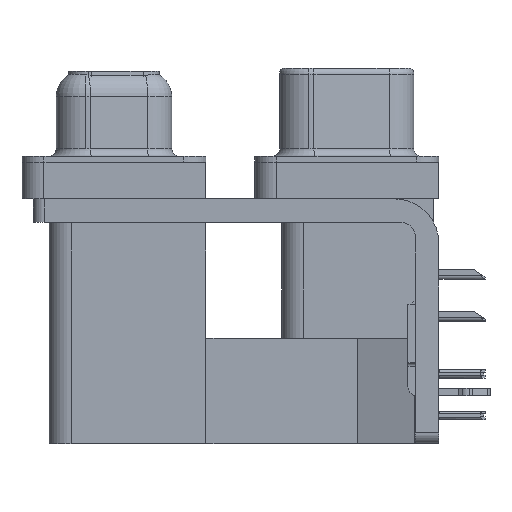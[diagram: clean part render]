
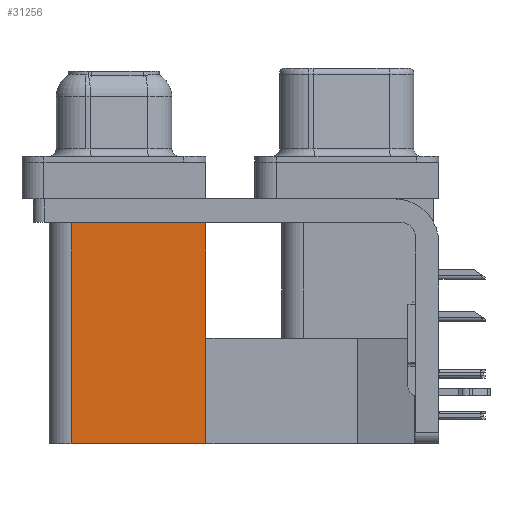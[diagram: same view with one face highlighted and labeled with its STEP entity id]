
A CAD part, left-side view. The second image highlights one B-rep face of the part: STEP entity #31256.
In plain terms, the highlighted planar face has unit normal (-1, 0, 0).
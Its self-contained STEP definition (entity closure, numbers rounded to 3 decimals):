
#248 = AXIS2_PLACEMENT_3D ( 'NONE', #3886, #31192, #4079 ) ;
#544 = CARTESIAN_POINT ( 'NONE',  ( 3.79, 18.8, -19.2 ) ) ;
#741 = CARTESIAN_POINT ( 'NONE',  ( 3.79, 9.6, -2.5 ) ) ;
#758 = CARTESIAN_POINT ( 'NONE',  ( 3.79, 18.8, -2.5 ) ) ;
#1249 = VECTOR ( 'NONE', #10169, 1000. ) ;
#1375 = EDGE_CURVE ( 'NONE', #37500, #7549, #36709, .T. ) ;
#1612 = EDGE_CURVE ( 'NONE', #25228, #7549, #31008, .T. ) ;
#3884 = DIRECTION ( 'NONE',  ( 0., 1., 0. ) ) ;
#3886 = CARTESIAN_POINT ( 'NONE',  ( 3.79, 9.6, -19.2 ) ) ;
#4079 = DIRECTION ( 'NONE',  ( 0., 1., 0. ) ) ;
#6852 = FACE_OUTER_BOUND ( 'NONE', #30425, .T. ) ;
#7549 = VERTEX_POINT ( 'NONE', #758 ) ;
#10169 = DIRECTION ( 'NONE',  ( 0., 0., 1. ) ) ;
#12331 = VECTOR ( 'NONE', #37831, 1000. ) ;
#12776 = ORIENTED_EDGE ( 'NONE', *, *, #1375, .F. ) ;
#14203 = CARTESIAN_POINT ( 'NONE',  ( 3.79, 9.6, -19.2 ) ) ;
#15921 = CARTESIAN_POINT ( 'NONE',  ( 3.79, 18.8, -19.2 ) ) ;
#16997 = VERTEX_POINT ( 'NONE', #14203 ) ;
#18748 = LINE ( 'NONE', #33981, #31999 ) ;
#19130 = DIRECTION ( 'NONE',  ( 0., 1., 0. ) ) ;
#22229 = ORIENTED_EDGE ( 'NONE', *, *, #36298, .F. ) ;
#23211 = ORIENTED_EDGE ( 'NONE', *, *, #27570, .T. ) ;
#25228 = VERTEX_POINT ( 'NONE', #37923 ) ;
#25776 = LINE ( 'NONE', #37448, #12331 ) ;
#27570 = EDGE_CURVE ( 'NONE', #16997, #25228, #25776, .T. ) ;
#30425 = EDGE_LOOP ( 'NONE', ( #32935, #12776, #22229, #23211 ) ) ;
#31008 = LINE ( 'NONE', #741, #32194 ) ;
#31192 = DIRECTION ( 'NONE',  ( 1., 0., 0. ) ) ;
#31256 = ADVANCED_FACE ( 'NONE', ( #6852 ), #37702, .F. ) ;
#31999 = VECTOR ( 'NONE', #19130, 1000. ) ;
#32194 = VECTOR ( 'NONE', #3884, 1000. ) ;
#32935 = ORIENTED_EDGE ( 'NONE', *, *, #1612, .T. ) ;
#33981 = CARTESIAN_POINT ( 'NONE',  ( 3.79, 9.6, -19.2 ) ) ;
#36298 = EDGE_CURVE ( 'NONE', #16997, #37500, #18748, .T. ) ;
#36709 = LINE ( 'NONE', #15921, #1249 ) ;
#37448 = CARTESIAN_POINT ( 'NONE',  ( 3.79, 9.6, -19.2 ) ) ;
#37500 = VERTEX_POINT ( 'NONE', #544 ) ;
#37702 = PLANE ( 'NONE',  #248 ) ;
#37831 = DIRECTION ( 'NONE',  ( 0., 0., 1. ) ) ;
#37923 = CARTESIAN_POINT ( 'NONE',  ( 3.79, 9.6, -2.5 ) ) ;
